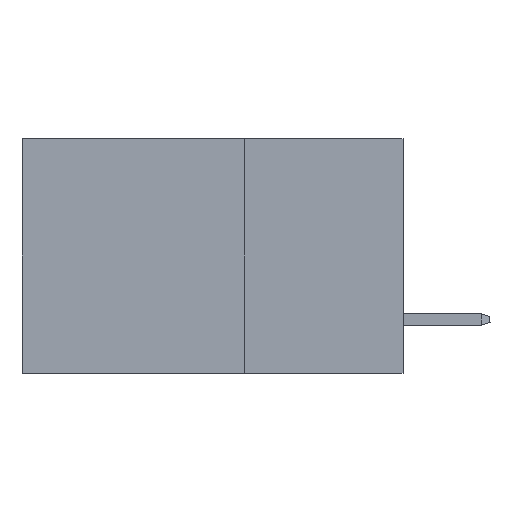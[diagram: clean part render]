
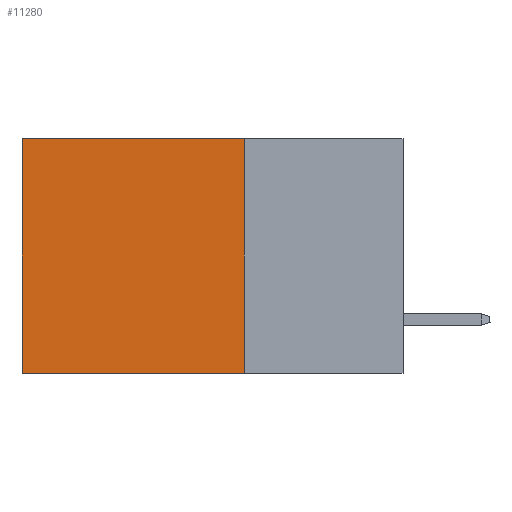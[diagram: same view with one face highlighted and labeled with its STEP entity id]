
A CAD part, left-side view. The second image highlights one B-rep face of the part: STEP entity #11280.
In plain terms, the highlighted planar face has unit normal (-1, 0, 0).
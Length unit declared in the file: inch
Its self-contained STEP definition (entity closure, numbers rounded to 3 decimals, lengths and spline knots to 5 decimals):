
#1447 = PLANE ( 'NONE',  #6771 ) ;
#3726 = EDGE_CURVE ( 'NONE', #42099, #34013, #23797, .T. ) ;
#4065 = LINE ( 'NONE', #28432, #6246 ) ;
#6246 = VECTOR ( 'NONE', #42652, 39.37008 ) ;
#6567 = ORIENTED_EDGE ( 'NONE', *, *, #16795, .F. ) ;
#6771 = AXIS2_PLACEMENT_3D ( 'NONE', #40226, #43045, #36279 ) ;
#6911 = LINE ( 'NONE', #39882, #44994 ) ;
#7677 = LINE ( 'NONE', #10694, #20700 ) ;
#8387 = VERTEX_POINT ( 'NONE', #17383 ) ;
#10694 = CARTESIAN_POINT ( 'NONE',  ( 0.2875, 0.25, 0. ) ) ;
#11280 = ADVANCED_FACE ( 'NONE', ( #29737 ), #1447, .F. ) ;
#15541 = CARTESIAN_POINT ( 'NONE',  ( 0.2875, 0.6, 0. ) ) ;
#16350 = CARTESIAN_POINT ( 'NONE',  ( 0.2875, 0.6, 0. ) ) ;
#16795 = EDGE_CURVE ( 'NONE', #8387, #34013, #4065, .T. ) ;
#16983 = ORIENTED_EDGE ( 'NONE', *, *, #30584, .T. ) ;
#17383 = CARTESIAN_POINT ( 'NONE',  ( 0.2875, 0.25, -0.37 ) ) ;
#19079 = VECTOR ( 'NONE', #37745, 39.37008 ) ;
#20586 = EDGE_CURVE ( 'NONE', #27660, #8387, #6911, .T. ) ;
#20700 = VECTOR ( 'NONE', #24852, 39.37008 ) ;
#23797 = LINE ( 'NONE', #16350, #19079 ) ;
#24852 = DIRECTION ( 'NONE',  ( 0., 1., 0. ) ) ;
#27660 = VERTEX_POINT ( 'NONE', #36602 ) ;
#28432 = CARTESIAN_POINT ( 'NONE',  ( 0.2875, 0.25, -0.37 ) ) ;
#28931 = CARTESIAN_POINT ( 'NONE',  ( 0.2875, 0.6, -0.37 ) ) ;
#29737 = FACE_OUTER_BOUND ( 'NONE', #32722, .T. ) ;
#30584 = EDGE_CURVE ( 'NONE', #27660, #42099, #7677, .T. ) ;
#32722 = EDGE_LOOP ( 'NONE', ( #41212, #6567, #40219, #16983 ) ) ;
#34013 = VERTEX_POINT ( 'NONE', #28931 ) ;
#36279 = DIRECTION ( 'NONE',  ( 0., 0., -1. ) ) ;
#36602 = CARTESIAN_POINT ( 'NONE',  ( 0.2875, 0.25, 0. ) ) ;
#37218 = DIRECTION ( 'NONE',  ( 0., 0., -1. ) ) ;
#37745 = DIRECTION ( 'NONE',  ( 0., 0., -1. ) ) ;
#39882 = CARTESIAN_POINT ( 'NONE',  ( 0.2875, 0.25, 0. ) ) ;
#40219 = ORIENTED_EDGE ( 'NONE', *, *, #20586, .F. ) ;
#40226 = CARTESIAN_POINT ( 'NONE',  ( 0.2875, 0.25, 0. ) ) ;
#41212 = ORIENTED_EDGE ( 'NONE', *, *, #3726, .T. ) ;
#42099 = VERTEX_POINT ( 'NONE', #15541 ) ;
#42652 = DIRECTION ( 'NONE',  ( 0., 1., 0. ) ) ;
#43045 = DIRECTION ( 'NONE',  ( 1., 0., 0. ) ) ;
#44994 = VECTOR ( 'NONE', #37218, 39.37008 ) ;
